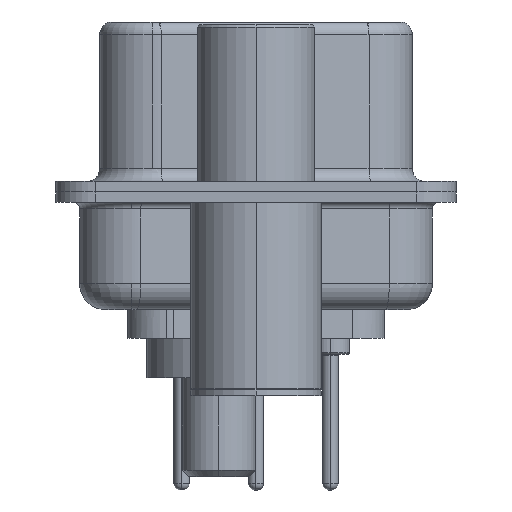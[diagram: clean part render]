
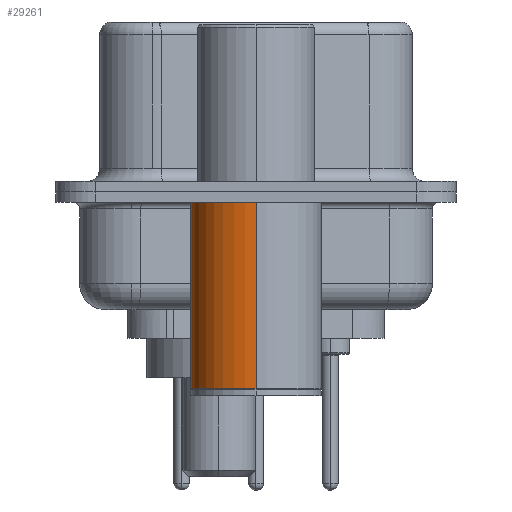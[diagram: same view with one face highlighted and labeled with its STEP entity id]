
A CAD part, left-side view. The second image highlights one B-rep face of the part: STEP entity #29261.
In plain terms, the highlighted cylindrical face has radius 2.5 mm (diameter 5 mm), a partial arc.
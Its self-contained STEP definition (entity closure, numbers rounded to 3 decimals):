
#184 = FACE_OUTER_BOUND ( 'NONE', #26832, .T. ) ;
#363 = CARTESIAN_POINT ( 'NONE',  ( -2.5, 0., -7.525 ) ) ;
#1640 = DIRECTION ( 'NONE',  ( 1., 0., 0. ) ) ;
#1975 = ORIENTED_EDGE ( 'NONE', *, *, #28428, .F. ) ;
#3507 = CARTESIAN_POINT ( 'NONE',  ( 2.5, 0., -7.525 ) ) ;
#4602 = ORIENTED_EDGE ( 'NONE', *, *, #30116, .T. ) ;
#4736 = AXIS2_PLACEMENT_3D ( 'NONE', #12050, #29945, #14572 ) ;
#6713 = DIRECTION ( 'NONE',  ( 0., 0., 1. ) ) ;
#6735 = ORIENTED_EDGE ( 'NONE', *, *, #17066, .F. ) ;
#6880 = VERTEX_POINT ( 'NONE', #26496 ) ;
#7497 = VERTEX_POINT ( 'NONE', #17430 ) ;
#8528 = VERTEX_POINT ( 'NONE', #3507 ) ;
#9075 = VERTEX_POINT ( 'NONE', #363 ) ;
#11296 = VECTOR ( 'NONE', #6713, 1000. ) ;
#12050 = CARTESIAN_POINT ( 'NONE',  ( 0., 0., -0.4 ) ) ;
#13715 = AXIS2_PLACEMENT_3D ( 'NONE', #32468, #17110, #1640 ) ;
#14453 = DIRECTION ( 'NONE',  ( 1., 0., 0. ) ) ;
#14560 = CARTESIAN_POINT ( 'NONE',  ( 0., 0., 0.581 ) ) ;
#14572 = DIRECTION ( 'NONE',  ( 1., 0., 0. ) ) ;
#16094 = CARTESIAN_POINT ( 'NONE',  ( -2.5, 0., 0.581 ) ) ;
#17066 = EDGE_CURVE ( 'NONE', #8528, #6880, #30099, .T. ) ;
#17110 = DIRECTION ( 'NONE',  ( 0., 0., 1. ) ) ;
#17430 = CARTESIAN_POINT ( 'NONE',  ( -2.5, 0., -0.4 ) ) ;
#19190 = EDGE_CURVE ( 'NONE', #8528, #9075, #28775, .T. ) ;
#20014 = CYLINDRICAL_SURFACE ( 'NONE', #21787, 2.5 ) ;
#21787 = AXIS2_PLACEMENT_3D ( 'NONE', #14560, #22258, #14453 ) ;
#22258 = DIRECTION ( 'NONE',  ( 0., 0., 1. ) ) ;
#24676 = CARTESIAN_POINT ( 'NONE',  ( 2.5, 0., 0.581 ) ) ;
#26496 = CARTESIAN_POINT ( 'NONE',  ( 2.5, 0., -0.4 ) ) ;
#26832 = EDGE_LOOP ( 'NONE', ( #32239, #4602, #1975, #6735 ) ) ;
#27139 = VECTOR ( 'NONE', #31443, 1000. ) ;
#27941 = LINE ( 'NONE', #16094, #27139 ) ;
#28428 = EDGE_CURVE ( 'NONE', #6880, #7497, #32432, .T. ) ;
#28775 = CIRCLE ( 'NONE', #13715, 2.5 ) ;
#29261 = ADVANCED_FACE ( 'NONE', ( #184 ), #20014, .T. ) ;
#29945 = DIRECTION ( 'NONE',  ( 0., 0., 1. ) ) ;
#30099 = LINE ( 'NONE', #24676, #11296 ) ;
#30116 = EDGE_CURVE ( 'NONE', #9075, #7497, #27941, .T. ) ;
#31443 = DIRECTION ( 'NONE',  ( 0., 0., 1. ) ) ;
#32239 = ORIENTED_EDGE ( 'NONE', *, *, #19190, .T. ) ;
#32432 = CIRCLE ( 'NONE', #4736, 2.5 ) ;
#32468 = CARTESIAN_POINT ( 'NONE',  ( 0., 0., -7.525 ) ) ;
